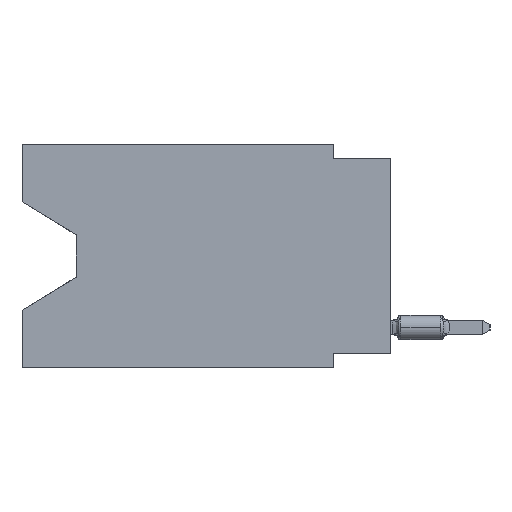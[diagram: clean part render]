
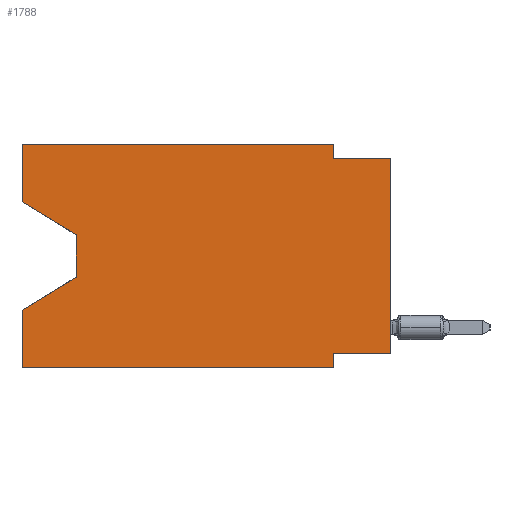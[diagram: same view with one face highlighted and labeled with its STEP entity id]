
A CAD part, left-side view. The second image highlights one B-rep face of the part: STEP entity #1788.
In plain terms, the highlighted planar face has unit normal (-1, 0, 0).
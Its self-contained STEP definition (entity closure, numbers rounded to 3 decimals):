
#1030 = ORIENTED_EDGE ( 'NONE', *, *, #36184, .T. ) ;
#1788 = ADVANCED_FACE ( 'NONE', ( #29262 ), #8987, .F. ) ;
#1802 = ORIENTED_EDGE ( 'NONE', *, *, #17186, .F. ) ;
#2204 = EDGE_CURVE ( 'NONE', #18515, #30168, #20328, .T. ) ;
#2371 = LINE ( 'NONE', #13908, #18694 ) ;
#2510 = DIRECTION ( 'NONE',  ( 0., 1., 0. ) ) ;
#2955 = CARTESIAN_POINT ( 'NONE',  ( 0., 0., -0.635 ) ) ;
#3115 = DIRECTION ( 'NONE',  ( 0., 0., -1. ) ) ;
#3672 = CARTESIAN_POINT ( 'NONE',  ( 0., 16.383, -9.906 ) ) ;
#3889 = VERTEX_POINT ( 'NONE', #22867 ) ;
#4142 = CARTESIAN_POINT ( 'NONE',  ( 0., 16.383, -2.546 ) ) ;
#4813 = VERTEX_POINT ( 'NONE', #36521 ) ;
#4841 = DIRECTION ( 'NONE',  ( 0., 0.855, -0.519 ) ) ;
#5114 = LINE ( 'NONE', #22343, #28142 ) ;
#5459 = LINE ( 'NONE', #10945, #20178 ) ;
#5732 = CARTESIAN_POINT ( 'NONE',  ( 0., 0., -9.271 ) ) ;
#6079 = EDGE_CURVE ( 'NONE', #31508, #3889, #5114, .T. ) ;
#6546 = CARTESIAN_POINT ( 'NONE',  ( 0., 13.97, -5.893 ) ) ;
#7101 = ORIENTED_EDGE ( 'NONE', *, *, #21847, .T. ) ;
#7493 = LINE ( 'NONE', #36496, #27629 ) ;
#8116 = DIRECTION ( 'NONE',  ( 0., 0., 1. ) ) ;
#8361 = DIRECTION ( 'NONE',  ( 0., 0., -1. ) ) ;
#8533 = DIRECTION ( 'NONE',  ( 0., -1., 0. ) ) ;
#8534 = DIRECTION ( 'NONE',  ( 0., 0., -1. ) ) ;
#8729 = CARTESIAN_POINT ( 'NONE',  ( 0., 13.97, -4.013 ) ) ;
#8750 = LINE ( 'NONE', #20324, #25128 ) ;
#8803 = CARTESIAN_POINT ( 'NONE',  ( 0., 16.383, 0. ) ) ;
#8987 = PLANE ( 'NONE',  #34493 ) ;
#10296 = VECTOR ( 'NONE', #3115, 1000. ) ;
#10793 = EDGE_CURVE ( 'NONE', #18515, #33063, #5459, .T. ) ;
#10913 = VECTOR ( 'NONE', #2510, 1000. ) ;
#10945 = CARTESIAN_POINT ( 'NONE',  ( 0., 0., 0. ) ) ;
#11285 = VERTEX_POINT ( 'NONE', #6546 ) ;
#11594 = ORIENTED_EDGE ( 'NONE', *, *, #10793, .T. ) ;
#12096 = VERTEX_POINT ( 'NONE', #15752 ) ;
#12587 = ORIENTED_EDGE ( 'NONE', *, *, #6079, .F. ) ;
#13397 = VECTOR ( 'NONE', #8534, 1000. ) ;
#13553 = CARTESIAN_POINT ( 'NONE',  ( 0., 2.54, -9.271 ) ) ;
#13776 = EDGE_CURVE ( 'NONE', #32512, #20908, #29062, .T. ) ;
#13908 = CARTESIAN_POINT ( 'NONE',  ( 0., 16.383, 0. ) ) ;
#14189 = CARTESIAN_POINT ( 'NONE',  ( 0., 0., -9.271 ) ) ;
#14351 = EDGE_CURVE ( 'NONE', #32512, #4813, #2371, .T. ) ;
#14918 = ORIENTED_EDGE ( 'NONE', *, *, #35624, .T. ) ;
#15616 = ORIENTED_EDGE ( 'NONE', *, *, #27361, .F. ) ;
#15752 = CARTESIAN_POINT ( 'NONE',  ( 0., 16.383, -2.546 ) ) ;
#16267 = VERTEX_POINT ( 'NONE', #37147 ) ;
#17124 = CARTESIAN_POINT ( 'NONE',  ( 0., 16.383, 0. ) ) ;
#17186 = EDGE_CURVE ( 'NONE', #3889, #16267, #32492, .T. ) ;
#17704 = CARTESIAN_POINT ( 'NONE',  ( 0., 2.54, 0. ) ) ;
#17841 = ORIENTED_EDGE ( 'NONE', *, *, #25649, .F. ) ;
#18515 = VERTEX_POINT ( 'NONE', #14189 ) ;
#18694 = VECTOR ( 'NONE', #27946, 1000. ) ;
#19141 = VECTOR ( 'NONE', #32757, 1000. ) ;
#19346 = EDGE_CURVE ( 'NONE', #12096, #31508, #8750, .T. ) ;
#19377 = ORIENTED_EDGE ( 'NONE', *, *, #19346, .F. ) ;
#19907 = CARTESIAN_POINT ( 'NONE',  ( 0., 0., -0.635 ) ) ;
#20178 = VECTOR ( 'NONE', #8116, 1000. ) ;
#20324 = CARTESIAN_POINT ( 'NONE',  ( 0., 16.383, 0. ) ) ;
#20328 = LINE ( 'NONE', #5732, #10913 ) ;
#20908 = VERTEX_POINT ( 'NONE', #37405 ) ;
#21205 = LINE ( 'NONE', #4142, #19141 ) ;
#21847 = EDGE_CURVE ( 'NONE', #35730, #11285, #33941, .T. ) ;
#22161 = DIRECTION ( 'NONE',  ( 0., -1., 0. ) ) ;
#22172 = ORIENTED_EDGE ( 'NONE', *, *, #14351, .F. ) ;
#22343 = CARTESIAN_POINT ( 'NONE',  ( 0., 16.383, 0. ) ) ;
#22684 = VECTOR ( 'NONE', #8533, 1000. ) ;
#22867 = CARTESIAN_POINT ( 'NONE',  ( 0., 2.54, 0. ) ) ;
#23952 = DIRECTION ( 'NONE',  ( 0., -1., 0. ) ) ;
#24306 = VECTOR ( 'NONE', #8361, 1000. ) ;
#24484 = LINE ( 'NONE', #25614, #24306 ) ;
#25128 = VECTOR ( 'NONE', #31871, 1000. ) ;
#25234 = LINE ( 'NONE', #19907, #22684 ) ;
#25614 = CARTESIAN_POINT ( 'NONE',  ( 0., 2.54, -9.906 ) ) ;
#25649 = EDGE_CURVE ( 'NONE', #16267, #33063, #25234, .T. ) ;
#26702 = EDGE_LOOP ( 'NONE', ( #14918, #7101, #1030, #22172, #26763, #15616, #29069, #11594, #17841, #1802, #12587, #19377 ) ) ;
#26763 = ORIENTED_EDGE ( 'NONE', *, *, #13776, .T. ) ;
#27361 = EDGE_CURVE ( 'NONE', #30168, #20908, #24484, .T. ) ;
#27629 = VECTOR ( 'NONE', #4841, 1000. ) ;
#27946 = DIRECTION ( 'NONE',  ( 0., 0., 1. ) ) ;
#28142 = VECTOR ( 'NONE', #22161, 1000. ) ;
#28889 = DIRECTION ( 'NONE',  ( 0., 0., -1. ) ) ;
#29062 = LINE ( 'NONE', #3672, #31377 ) ;
#29069 = ORIENTED_EDGE ( 'NONE', *, *, #2204, .F. ) ;
#29262 = FACE_OUTER_BOUND ( 'NONE', #26702, .T. ) ;
#30168 = VERTEX_POINT ( 'NONE', #13553 ) ;
#31377 = VECTOR ( 'NONE', #23952, 1000. ) ;
#31508 = VERTEX_POINT ( 'NONE', #17124 ) ;
#31871 = DIRECTION ( 'NONE',  ( 0., 0., 1. ) ) ;
#32492 = LINE ( 'NONE', #17704, #10296 ) ;
#32512 = VERTEX_POINT ( 'NONE', #35920 ) ;
#32757 = DIRECTION ( 'NONE',  ( 0., -0.855, -0.519 ) ) ;
#33063 = VERTEX_POINT ( 'NONE', #2955 ) ;
#33941 = LINE ( 'NONE', #8729, #13397 ) ;
#34493 = AXIS2_PLACEMENT_3D ( 'NONE', #8803, #34581, #28889 ) ;
#34581 = DIRECTION ( 'NONE',  ( 1., 0., 0. ) ) ;
#35608 = CARTESIAN_POINT ( 'NONE',  ( 0., 13.97, -4.013 ) ) ;
#35624 = EDGE_CURVE ( 'NONE', #12096, #35730, #21205, .T. ) ;
#35730 = VERTEX_POINT ( 'NONE', #35608 ) ;
#35920 = CARTESIAN_POINT ( 'NONE',  ( 0., 16.383, -9.906 ) ) ;
#36184 = EDGE_CURVE ( 'NONE', #11285, #4813, #7493, .T. ) ;
#36496 = CARTESIAN_POINT ( 'NONE',  ( 0., 13.97, -5.893 ) ) ;
#36521 = CARTESIAN_POINT ( 'NONE',  ( 0., 16.383, -7.36 ) ) ;
#37147 = CARTESIAN_POINT ( 'NONE',  ( 0., 2.54, -0.635 ) ) ;
#37405 = CARTESIAN_POINT ( 'NONE',  ( 0., 2.54, -9.906 ) ) ;
